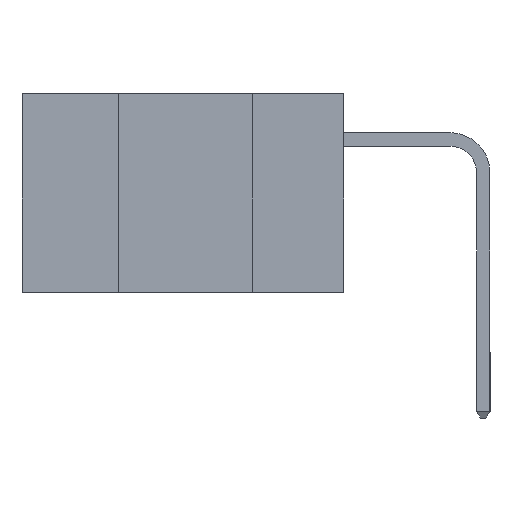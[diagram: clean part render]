
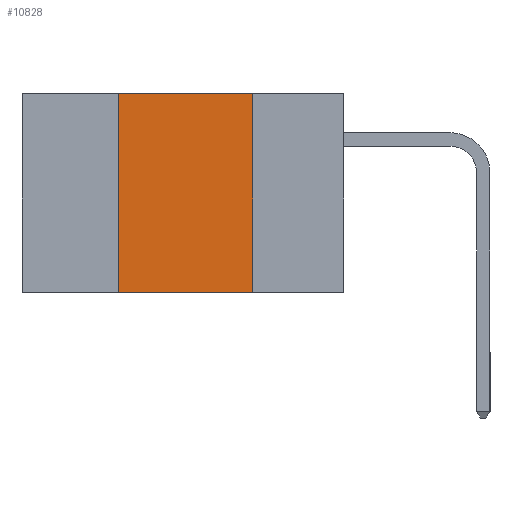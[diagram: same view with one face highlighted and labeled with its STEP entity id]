
A CAD part, left-side view. The second image highlights one B-rep face of the part: STEP entity #10828.
In plain terms, the highlighted planar face has unit normal (-1, 0, 0).
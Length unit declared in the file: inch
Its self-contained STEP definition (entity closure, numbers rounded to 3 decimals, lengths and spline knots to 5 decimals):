
#1590 = DIRECTION ( 'NONE',  ( 1., 0., 0. ) ) ;
#1684 = PLANE ( 'NONE',  #7200 ) ;
#1761 = ORIENTED_EDGE ( 'NONE', *, *, #10794, .F. ) ;
#2176 = ORIENTED_EDGE ( 'NONE', *, *, #12189, .T. ) ;
#2394 = LINE ( 'NONE', #10650, #10817 ) ;
#2514 = VECTOR ( 'NONE', #14181, 39.37008 ) ;
#2620 = DIRECTION ( 'NONE',  ( 0., 0., 1. ) ) ;
#2628 = CARTESIAN_POINT ( 'NONE',  ( 0., 0.17, 0. ) ) ;
#2649 = FACE_OUTER_BOUND ( 'NONE', #8354, .T. ) ;
#2920 = EDGE_CURVE ( 'NONE', #6054, #14584, #2394, .T. ) ;
#3659 = CARTESIAN_POINT ( 'NONE',  ( 0., 0.6, -0.37 ) ) ;
#4143 = VECTOR ( 'NONE', #11046, 39.37008 ) ;
#5116 = VERTEX_POINT ( 'NONE', #7637 ) ;
#5626 = CARTESIAN_POINT ( 'NONE',  ( 0., 0.42, 0. ) ) ;
#6054 = VERTEX_POINT ( 'NONE', #5626 ) ;
#6354 = CARTESIAN_POINT ( 'NONE',  ( 0., 0.42, 0. ) ) ;
#6391 = ORIENTED_EDGE ( 'NONE', *, *, #7083, .F. ) ;
#7083 = EDGE_CURVE ( 'NONE', #13329, #6054, #14718, .T. ) ;
#7200 = AXIS2_PLACEMENT_3D ( 'NONE', #12432, #1590, #14674 ) ;
#7637 = CARTESIAN_POINT ( 'NONE',  ( 0., 0.17, -0.37 ) ) ;
#8036 = CARTESIAN_POINT ( 'NONE',  ( 0., 0.17, 0. ) ) ;
#8354 = EDGE_LOOP ( 'NONE', ( #1761, #11666, #6391, #2176 ) ) ;
#10270 = CARTESIAN_POINT ( 'NONE',  ( 0., 0.42, -0.37 ) ) ;
#10494 = LINE ( 'NONE', #2628, #4143 ) ;
#10650 = CARTESIAN_POINT ( 'NONE',  ( 0., 0.6, 0. ) ) ;
#10794 = EDGE_CURVE ( 'NONE', #14584, #5116, #10494, .T. ) ;
#10817 = VECTOR ( 'NONE', #14549, 39.37008 ) ;
#10828 = ADVANCED_FACE ( 'NONE', ( #2649 ), #1684, .F. ) ;
#11046 = DIRECTION ( 'NONE',  ( 0., 0., -1. ) ) ;
#11666 = ORIENTED_EDGE ( 'NONE', *, *, #2920, .F. ) ;
#12189 = EDGE_CURVE ( 'NONE', #13329, #5116, #13891, .T. ) ;
#12432 = CARTESIAN_POINT ( 'NONE',  ( 0., 0.6, 0. ) ) ;
#13329 = VERTEX_POINT ( 'NONE', #10270 ) ;
#13891 = LINE ( 'NONE', #3659, #2514 ) ;
#14181 = DIRECTION ( 'NONE',  ( 0., -1., 0. ) ) ;
#14549 = DIRECTION ( 'NONE',  ( 0., -1., 0. ) ) ;
#14584 = VERTEX_POINT ( 'NONE', #8036 ) ;
#14674 = DIRECTION ( 'NONE',  ( 0., 0., -1. ) ) ;
#14718 = LINE ( 'NONE', #6354, #14903 ) ;
#14903 = VECTOR ( 'NONE', #2620, 39.37008 ) ;
